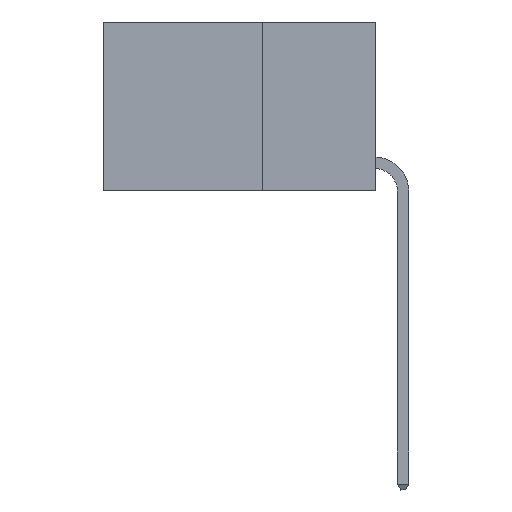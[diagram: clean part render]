
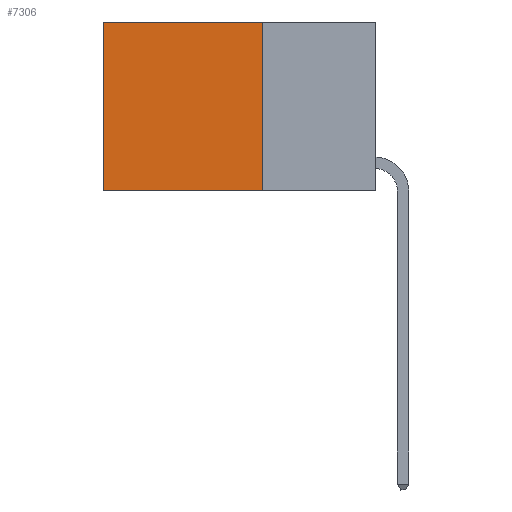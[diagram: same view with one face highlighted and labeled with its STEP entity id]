
A CAD part, left-side view. The second image highlights one B-rep face of the part: STEP entity #7306.
In plain terms, the highlighted planar face has unit normal (-1, 0, 0).
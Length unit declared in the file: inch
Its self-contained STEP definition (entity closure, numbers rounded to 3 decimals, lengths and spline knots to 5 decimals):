
#29 = VERTEX_POINT ( 'NONE', #8397 ) ;
#1073 = EDGE_CURVE ( 'NONE', #7376, #29, #9492, .T. ) ;
#1077 = DIRECTION ( 'NONE',  ( 0., 1., 0. ) ) ;
#1471 = DIRECTION ( 'NONE',  ( 1., 0., 0. ) ) ;
#1762 = VECTOR ( 'NONE', #8695, 39.37008 ) ;
#2172 = CARTESIAN_POINT ( 'NONE',  ( 0.2625, 0.6, 0. ) ) ;
#2227 = ORIENTED_EDGE ( 'NONE', *, *, #8328, .F. ) ;
#2261 = LINE ( 'NONE', #9641, #1762 ) ;
#2349 = CARTESIAN_POINT ( 'NONE',  ( 0.2625, 0.6, 0. ) ) ;
#2542 = VECTOR ( 'NONE', #8959, 39.37008 ) ;
#3250 = LINE ( 'NONE', #5121, #2542 ) ;
#3433 = AXIS2_PLACEMENT_3D ( 'NONE', #10531, #1471, #4266 ) ;
#4146 = FACE_OUTER_BOUND ( 'NONE', #11679, .T. ) ;
#4266 = DIRECTION ( 'NONE',  ( 0., 0., -1. ) ) ;
#5121 = CARTESIAN_POINT ( 'NONE',  ( 0.2625, 0.25, 0. ) ) ;
#5324 = VERTEX_POINT ( 'NONE', #11692 ) ;
#6357 = VERTEX_POINT ( 'NONE', #9680 ) ;
#6504 = CARTESIAN_POINT ( 'NONE',  ( 0.2625, 0.25, -0.37 ) ) ;
#6628 = LINE ( 'NONE', #6504, #7145 ) ;
#7145 = VECTOR ( 'NONE', #1077, 39.37008 ) ;
#7194 = ORIENTED_EDGE ( 'NONE', *, *, #1073, .T. ) ;
#7306 = ADVANCED_FACE ( 'NONE', ( #4146 ), #10418, .F. ) ;
#7376 = VERTEX_POINT ( 'NONE', #2172 ) ;
#7831 = VECTOR ( 'NONE', #8779, 39.37008 ) ;
#8328 = EDGE_CURVE ( 'NONE', #5324, #6357, #2261, .T. ) ;
#8397 = CARTESIAN_POINT ( 'NONE',  ( 0.2625, 0.6, -0.37 ) ) ;
#8695 = DIRECTION ( 'NONE',  ( 0., 0., -1. ) ) ;
#8779 = DIRECTION ( 'NONE',  ( 0., 0., -1. ) ) ;
#8950 = ORIENTED_EDGE ( 'NONE', *, *, #10667, .T. ) ;
#8959 = DIRECTION ( 'NONE',  ( 0., 1., 0. ) ) ;
#9492 = LINE ( 'NONE', #2349, #7831 ) ;
#9641 = CARTESIAN_POINT ( 'NONE',  ( 0.2625, 0.25, 0. ) ) ;
#9680 = CARTESIAN_POINT ( 'NONE',  ( 0.2625, 0.25, -0.37 ) ) ;
#9903 = ORIENTED_EDGE ( 'NONE', *, *, #9933, .F. ) ;
#9933 = EDGE_CURVE ( 'NONE', #6357, #29, #6628, .T. ) ;
#10418 = PLANE ( 'NONE',  #3433 ) ;
#10531 = CARTESIAN_POINT ( 'NONE',  ( 0.2625, 0.25, 0. ) ) ;
#10667 = EDGE_CURVE ( 'NONE', #5324, #7376, #3250, .T. ) ;
#11679 = EDGE_LOOP ( 'NONE', ( #7194, #9903, #2227, #8950 ) ) ;
#11692 = CARTESIAN_POINT ( 'NONE',  ( 0.2625, 0.25, 0. ) ) ;
